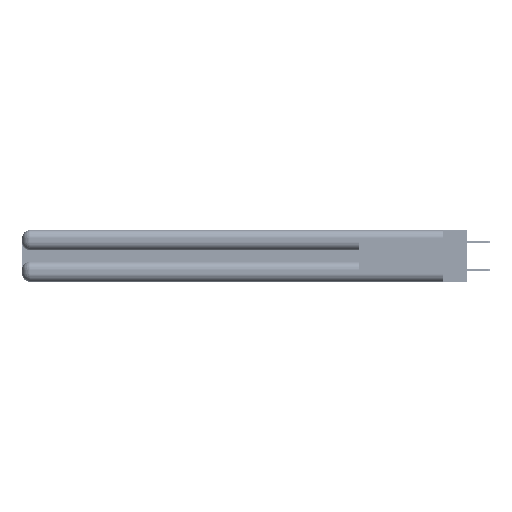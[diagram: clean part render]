
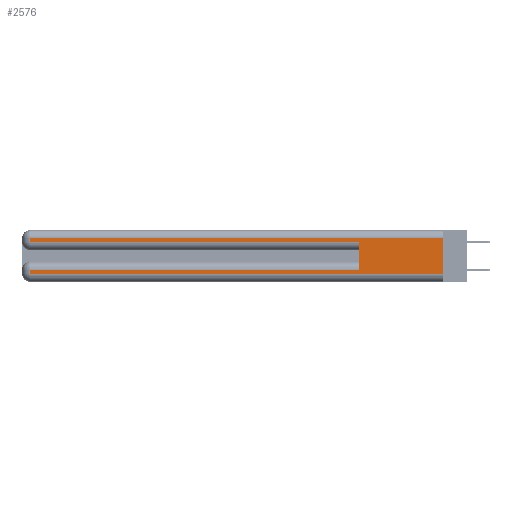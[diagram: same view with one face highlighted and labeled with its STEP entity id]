
A CAD part, left-side view. The second image highlights one B-rep face of the part: STEP entity #2576.
In plain terms, the highlighted planar face has unit normal (-1, 0, 0).
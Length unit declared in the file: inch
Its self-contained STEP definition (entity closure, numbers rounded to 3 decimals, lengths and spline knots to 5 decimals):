
#2490 = LINE ( 'NONE', #36935, #46588 ) ;
#2576 = ADVANCED_FACE ( 'NONE', ( #35013 ), #54327, .F. ) ;
#2837 = LINE ( 'NONE', #50778, #24237 ) ;
#3260 = DIRECTION ( 'NONE',  ( 1., 0., 0. ) ) ;
#4087 = ORIENTED_EDGE ( 'NONE', *, *, #32428, .T. ) ;
#7684 = LINE ( 'NONE', #28118, #39094 ) ;
#9437 = DIRECTION ( 'NONE',  ( 0., 1., 0. ) ) ;
#10029 = VECTOR ( 'NONE', #46956, 39.37008 ) ;
#10259 = VERTEX_POINT ( 'NONE', #52843 ) ;
#10903 = CARTESIAN_POINT ( 'NONE',  ( 0., 2.94, 0.085 ) ) ;
#12319 = ORIENTED_EDGE ( 'NONE', *, *, #13127, .F. ) ;
#13127 = EDGE_CURVE ( 'NONE', #48659, #22656, #15330, .T. ) ;
#13981 = EDGE_CURVE ( 'NONE', #14265, #22656, #2490, .T. ) ;
#14016 = VECTOR ( 'NONE', #52191, 39.37008 ) ;
#14265 = VERTEX_POINT ( 'NONE', #51351 ) ;
#15259 = DIRECTION ( 'NONE',  ( 0., 0., -1. ) ) ;
#15330 = LINE ( 'NONE', #18136, #14016 ) ;
#16505 = LINE ( 'NONE', #45026, #53138 ) ;
#17139 = CARTESIAN_POINT ( 'NONE',  ( 0., 0., 0.31 ) ) ;
#17201 = LINE ( 'NONE', #34998, #51164 ) ;
#18027 = EDGE_CURVE ( 'NONE', #38733, #23577, #2837, .T. ) ;
#18136 = CARTESIAN_POINT ( 'NONE',  ( 0., 0., 0.37 ) ) ;
#19077 = ORIENTED_EDGE ( 'NONE', *, *, #30110, .T. ) ;
#20787 = LINE ( 'NONE', #27888, #42194 ) ;
#22656 = VERTEX_POINT ( 'NONE', #37515 ) ;
#23577 = VERTEX_POINT ( 'NONE', #26030 ) ;
#23748 = DIRECTION ( 'NONE',  ( 0., 0., 1. ) ) ;
#24237 = VECTOR ( 'NONE', #55056, 39.37008 ) ;
#26030 = CARTESIAN_POINT ( 'NONE',  ( 0., 2.94, 0.285 ) ) ;
#27888 = CARTESIAN_POINT ( 'NONE',  ( 0., 0., 0.285 ) ) ;
#28118 = CARTESIAN_POINT ( 'NONE',  ( 0., 2.94, 0.37 ) ) ;
#28846 = CARTESIAN_POINT ( 'NONE',  ( 0., 0., 0.37 ) ) ;
#30110 = EDGE_CURVE ( 'NONE', #10259, #37090, #17201, .T. ) ;
#30361 = EDGE_CURVE ( 'NONE', #10259, #53283, #16505, .T. ) ;
#32185 = DIRECTION ( 'NONE',  ( 0., -1., 0. ) ) ;
#32258 = AXIS2_PLACEMENT_3D ( 'NONE', #28846, #3260, #33156 ) ;
#32428 = EDGE_CURVE ( 'NONE', #37090, #14265, #7684, .T. ) ;
#33156 = DIRECTION ( 'NONE',  ( 0., 0., -1. ) ) ;
#34998 = CARTESIAN_POINT ( 'NONE',  ( 0., 0., 0.085 ) ) ;
#35013 = FACE_OUTER_BOUND ( 'NONE', #45243, .T. ) ;
#35537 = ORIENTED_EDGE ( 'NONE', *, *, #30361, .F. ) ;
#36935 = CARTESIAN_POINT ( 'NONE',  ( 0., 0., 0.06 ) ) ;
#37090 = VERTEX_POINT ( 'NONE', #10903 ) ;
#37515 = CARTESIAN_POINT ( 'NONE',  ( 0., 0., 0.06 ) ) ;
#38733 = VERTEX_POINT ( 'NONE', #39134 ) ;
#39045 = ORIENTED_EDGE ( 'NONE', *, *, #44336, .T. ) ;
#39094 = VECTOR ( 'NONE', #15259, 39.37008 ) ;
#39134 = CARTESIAN_POINT ( 'NONE',  ( 0., 2.94, 0.31 ) ) ;
#39403 = CARTESIAN_POINT ( 'NONE',  ( 0., 0., 0.31 ) ) ;
#41373 = LINE ( 'NONE', #17139, #10029 ) ;
#42194 = VECTOR ( 'NONE', #32185, 39.37008 ) ;
#44336 = EDGE_CURVE ( 'NONE', #48659, #38733, #41373, .T. ) ;
#45026 = CARTESIAN_POINT ( 'NONE',  ( 0., 0.6, 0.145 ) ) ;
#45243 = EDGE_LOOP ( 'NONE', ( #12319, #39045, #47835, #52897, #35537, #19077, #4087, #45786 ) ) ;
#45786 = ORIENTED_EDGE ( 'NONE', *, *, #13981, .T. ) ;
#46588 = VECTOR ( 'NONE', #53971, 39.37008 ) ;
#46956 = DIRECTION ( 'NONE',  ( 0., 1., 0. ) ) ;
#47835 = ORIENTED_EDGE ( 'NONE', *, *, #18027, .T. ) ;
#48659 = VERTEX_POINT ( 'NONE', #39403 ) ;
#48748 = CARTESIAN_POINT ( 'NONE',  ( 0., 0.6, 0.285 ) ) ;
#50778 = CARTESIAN_POINT ( 'NONE',  ( 0., 2.94, 0.37 ) ) ;
#51164 = VECTOR ( 'NONE', #9437, 39.37008 ) ;
#51351 = CARTESIAN_POINT ( 'NONE',  ( 0., 2.94, 0.06 ) ) ;
#52191 = DIRECTION ( 'NONE',  ( 0., 0., -1. ) ) ;
#52843 = CARTESIAN_POINT ( 'NONE',  ( 0., 0.6, 0.085 ) ) ;
#52897 = ORIENTED_EDGE ( 'NONE', *, *, #54873, .T. ) ;
#53138 = VECTOR ( 'NONE', #23748, 39.37008 ) ;
#53283 = VERTEX_POINT ( 'NONE', #48748 ) ;
#53971 = DIRECTION ( 'NONE',  ( 0., -1., 0. ) ) ;
#54327 = PLANE ( 'NONE',  #32258 ) ;
#54873 = EDGE_CURVE ( 'NONE', #23577, #53283, #20787, .T. ) ;
#55056 = DIRECTION ( 'NONE',  ( 0., 0., -1. ) ) ;
